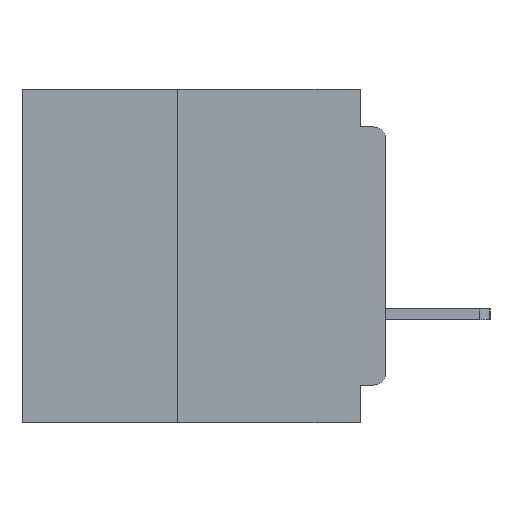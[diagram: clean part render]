
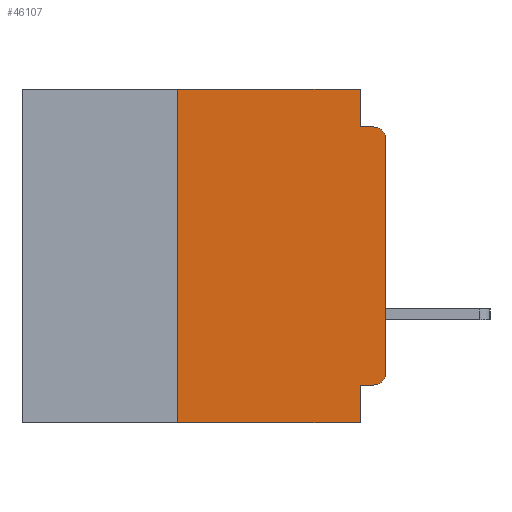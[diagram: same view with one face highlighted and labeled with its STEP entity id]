
A CAD part, left-side view. The second image highlights one B-rep face of the part: STEP entity #46107.
In plain terms, the highlighted planar face has unit normal (-1, 0, 0).
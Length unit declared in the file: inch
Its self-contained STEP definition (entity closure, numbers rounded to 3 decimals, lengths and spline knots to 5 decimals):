
#193 = DIRECTION ( 'NONE',  ( 0., 0., 1. ) ) ;
#612 = CARTESIAN_POINT ( 'NONE',  ( 0., 0.031, 0. ) ) ;
#2244 = ORIENTED_EDGE ( 'NONE', *, *, #7598, .F. ) ;
#3392 = ORIENTED_EDGE ( 'NONE', *, *, #14517, .T. ) ;
#3862 = ORIENTED_EDGE ( 'NONE', *, *, #51342, .F. ) ;
#3929 = VERTEX_POINT ( 'NONE', #34089 ) ;
#4721 = CARTESIAN_POINT ( 'NONE',  ( 0., 0., 0. ) ) ;
#4827 = DIRECTION ( 'NONE',  ( 0., -1., 0. ) ) ;
#5402 = FACE_OUTER_BOUND ( 'NONE', #52450, .T. ) ;
#5897 = VERTEX_POINT ( 'NONE', #19474 ) ;
#6943 = VERTEX_POINT ( 'NONE', #39419 ) ;
#6994 = VECTOR ( 'NONE', #4827, 39.37008 ) ;
#7504 = CARTESIAN_POINT ( 'NONE',  ( 0., 0.031, -0.045 ) ) ;
#7598 = EDGE_CURVE ( 'NONE', #5897, #14500, #8337, .T. ) ;
#8337 = LINE ( 'NONE', #30301, #6994 ) ;
#8998 = VERTEX_POINT ( 'NONE', #27002 ) ;
#9124 = CARTESIAN_POINT ( 'NONE',  ( 0., 0.015, -0.34 ) ) ;
#9542 = CARTESIAN_POINT ( 'NONE',  ( 0., 0.437, -0.4 ) ) ;
#10495 = PLANE ( 'NONE',  #46482 ) ;
#12215 = DIRECTION ( 'NONE',  ( -1., 0., 0. ) ) ;
#12902 = ORIENTED_EDGE ( 'NONE', *, *, #27916, .T. ) ;
#13046 = DIRECTION ( 'NONE',  ( 0., 0., -1. ) ) ;
#13383 = DIRECTION ( 'NONE',  ( 0., 0., -1. ) ) ;
#13800 = DIRECTION ( 'NONE',  ( 0., -1., 0. ) ) ;
#14500 = VERTEX_POINT ( 'NONE', #51011 ) ;
#14517 = EDGE_CURVE ( 'NONE', #14927, #41239, #33164, .T. ) ;
#14927 = VERTEX_POINT ( 'NONE', #28444 ) ;
#15725 = LINE ( 'NONE', #4721, #36995 ) ;
#15762 = EDGE_CURVE ( 'NONE', #41239, #8998, #15725, .T. ) ;
#18131 = LINE ( 'NONE', #9542, #39418 ) ;
#18196 = CARTESIAN_POINT ( 'NONE',  ( 0., 0.031, -0.355 ) ) ;
#19474 = CARTESIAN_POINT ( 'NONE',  ( 0., 0.25, 0. ) ) ;
#20797 = DIRECTION ( 'NONE',  ( 0., -1., 0. ) ) ;
#21018 = ORIENTED_EDGE ( 'NONE', *, *, #30690, .T. ) ;
#21108 = LINE ( 'NONE', #46011, #42306 ) ;
#21134 = CIRCLE ( 'NONE', #22282, 0.015 ) ;
#21405 = CARTESIAN_POINT ( 'NONE',  ( 0., 0.25, -0.4 ) ) ;
#21818 = DIRECTION ( 'NONE',  ( 0., 0., -1. ) ) ;
#22282 = AXIS2_PLACEMENT_3D ( 'NONE', #37701, #12215, #41938 ) ;
#23620 = VECTOR ( 'NONE', #13046, 39.37008 ) ;
#24771 = CARTESIAN_POINT ( 'NONE',  ( 0., 0.015, -0.045 ) ) ;
#26651 = LINE ( 'NONE', #33433, #36618 ) ;
#26742 = LINE ( 'NONE', #21405, #47762 ) ;
#27002 = CARTESIAN_POINT ( 'NONE',  ( 0., 0., -0.06 ) ) ;
#27624 = DIRECTION ( 'NONE',  ( 0., 0., -1. ) ) ;
#27916 = EDGE_CURVE ( 'NONE', #3929, #6943, #18131, .T. ) ;
#28327 = VERTEX_POINT ( 'NONE', #24771 ) ;
#28444 = CARTESIAN_POINT ( 'NONE',  ( 0., 0.015, -0.355 ) ) ;
#28463 = EDGE_CURVE ( 'NONE', #3929, #5897, #26742, .T. ) ;
#30301 = CARTESIAN_POINT ( 'NONE',  ( 0., 0.437, 0. ) ) ;
#30690 = EDGE_CURVE ( 'NONE', #8998, #28327, #21134, .T. ) ;
#31490 = EDGE_CURVE ( 'NONE', #45429, #6943, #36241, .T. ) ;
#33164 = CIRCLE ( 'NONE', #44661, 0.015 ) ;
#33433 = CARTESIAN_POINT ( 'NONE',  ( 0., 0., -0.045 ) ) ;
#34089 = CARTESIAN_POINT ( 'NONE',  ( 0., 0.25, -0.4 ) ) ;
#36209 = VERTEX_POINT ( 'NONE', #7504 ) ;
#36241 = LINE ( 'NONE', #46878, #23620 ) ;
#36618 = VECTOR ( 'NONE', #20797, 39.37008 ) ;
#36995 = VECTOR ( 'NONE', #38747, 39.37008 ) ;
#37112 = CARTESIAN_POINT ( 'NONE',  ( 0., 0., -0.34 ) ) ;
#37701 = CARTESIAN_POINT ( 'NONE',  ( 0., 0.015, -0.06 ) ) ;
#38747 = DIRECTION ( 'NONE',  ( 0., 0., 1. ) ) ;
#38876 = DIRECTION ( 'NONE',  ( -1., 0., 0. ) ) ;
#39174 = VECTOR ( 'NONE', #21818, 39.37008 ) ;
#39258 = ORIENTED_EDGE ( 'NONE', *, *, #48334, .F. ) ;
#39418 = VECTOR ( 'NONE', #13800, 39.37008 ) ;
#39419 = CARTESIAN_POINT ( 'NONE',  ( 0., 0.031, -0.4 ) ) ;
#40228 = CARTESIAN_POINT ( 'NONE',  ( 0., 0.437, 0. ) ) ;
#40481 = LINE ( 'NONE', #612, #39174 ) ;
#41239 = VERTEX_POINT ( 'NONE', #37112 ) ;
#41938 = DIRECTION ( 'NONE',  ( 0., 0., -1. ) ) ;
#42306 = VECTOR ( 'NONE', #50173, 39.37008 ) ;
#44413 = ORIENTED_EDGE ( 'NONE', *, *, #31490, .F. ) ;
#44661 = AXIS2_PLACEMENT_3D ( 'NONE', #9124, #38876, #13383 ) ;
#45429 = VERTEX_POINT ( 'NONE', #18196 ) ;
#46011 = CARTESIAN_POINT ( 'NONE',  ( 0., 0., -0.355 ) ) ;
#46107 = ADVANCED_FACE ( 'NONE', ( #5402 ), #10495, .F. ) ;
#46482 = AXIS2_PLACEMENT_3D ( 'NONE', #40228, #52693, #27624 ) ;
#46878 = CARTESIAN_POINT ( 'NONE',  ( 0., 0.031, -0.4 ) ) ;
#47762 = VECTOR ( 'NONE', #193, 39.37008 ) ;
#48334 = EDGE_CURVE ( 'NONE', #14927, #45429, #21108, .T. ) ;
#49206 = ORIENTED_EDGE ( 'NONE', *, *, #15762, .T. ) ;
#49703 = ORIENTED_EDGE ( 'NONE', *, *, #28463, .F. ) ;
#50173 = DIRECTION ( 'NONE',  ( 0., 1., 0. ) ) ;
#51011 = CARTESIAN_POINT ( 'NONE',  ( 0., 0.031, 0. ) ) ;
#51342 = EDGE_CURVE ( 'NONE', #36209, #28327, #26651, .T. ) ;
#52107 = EDGE_CURVE ( 'NONE', #14500, #36209, #40481, .T. ) ;
#52450 = EDGE_LOOP ( 'NONE', ( #49206, #21018, #3862, #53697, #2244, #49703, #12902, #44413, #39258, #3392 ) ) ;
#52693 = DIRECTION ( 'NONE',  ( 1., 0., 0. ) ) ;
#53697 = ORIENTED_EDGE ( 'NONE', *, *, #52107, .F. ) ;
